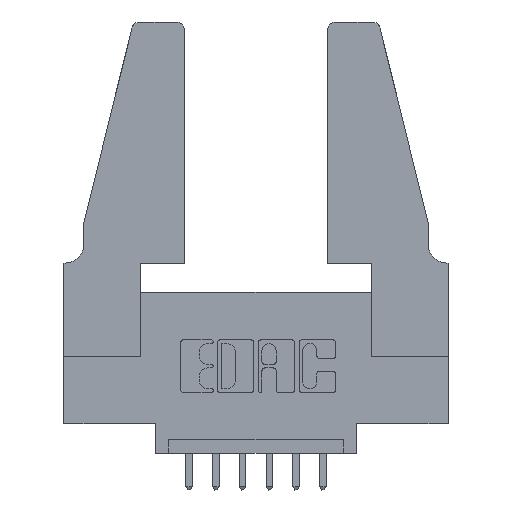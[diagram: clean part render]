
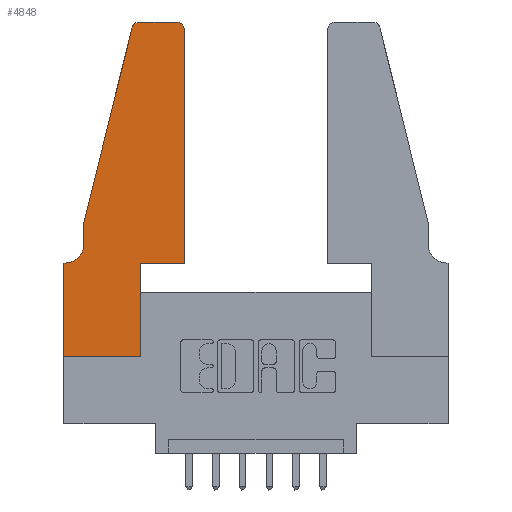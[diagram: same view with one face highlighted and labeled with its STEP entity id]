
A CAD part, top view. The second image highlights one B-rep face of the part: STEP entity #4848.
In plain terms, the highlighted planar face has unit normal (0, 0, 1).
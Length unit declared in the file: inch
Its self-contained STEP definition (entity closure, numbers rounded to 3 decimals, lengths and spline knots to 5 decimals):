
#144 = DIRECTION ( 'NONE',  ( 1., 0., 0. ) ) ;
#149 = VERTEX_POINT ( 'NONE', #6976 ) ;
#246 = ORIENTED_EDGE ( 'NONE', *, *, #10610, .T. ) ;
#506 = AXIS2_PLACEMENT_3D ( 'NONE', #6412, #2823, #144 ) ;
#513 = DIRECTION ( 'NONE',  ( -0.239, -0.971, 0. ) ) ;
#613 = LINE ( 'NONE', #10968, #7935 ) ;
#651 = EDGE_CURVE ( 'NONE', #149, #6248, #10727, .T. ) ;
#868 = AXIS2_PLACEMENT_3D ( 'NONE', #3825, #1192, #11094 ) ;
#982 = CARTESIAN_POINT ( 'NONE',  ( 0.4505, 1.22, 0.37 ) ) ;
#1148 = VERTEX_POINT ( 'NONE', #9154 ) ;
#1164 = VECTOR ( 'NONE', #2240, 39.37008 ) ;
#1192 = DIRECTION ( 'NONE',  ( 0., 0., -1. ) ) ;
#1407 = FACE_OUTER_BOUND ( 'NONE', #10970, .T. ) ;
#1627 = DIRECTION ( 'NONE',  ( 1., 0., 0. ) ) ;
#1780 = AXIS2_PLACEMENT_3D ( 'NONE', #10137, #6746, #8725 ) ;
#1840 = VECTOR ( 'NONE', #1627, 39.37008 ) ;
#2175 = LINE ( 'NONE', #9922, #9075 ) ;
#2212 = CARTESIAN_POINT ( 'NONE',  ( 0.0755, 0.42, 0.37 ) ) ;
#2240 = DIRECTION ( 'NONE',  ( 1., 0., 0. ) ) ;
#2250 = EDGE_CURVE ( 'NONE', #4102, #149, #9783, .T. ) ;
#2788 = EDGE_CURVE ( 'NONE', #1148, #4877, #2175, .T. ) ;
#2819 = VERTEX_POINT ( 'NONE', #5572 ) ;
#2823 = DIRECTION ( 'NONE',  ( 0., 0., 1. ) ) ;
#2910 = CARTESIAN_POINT ( 'NONE',  ( 0., 0.35, 0.37 ) ) ;
#2933 = EDGE_CURVE ( 'NONE', #4877, #8999, #613, .T. ) ;
#2944 = ORIENTED_EDGE ( 'NONE', *, *, #7547, .T. ) ;
#2983 = VERTEX_POINT ( 'NONE', #8595 ) ;
#3179 = CARTESIAN_POINT ( 'NONE',  ( 0.4505, 0.35, 0.37 ) ) ;
#3253 = CARTESIAN_POINT ( 'NONE',  ( 0.0755, 0.5, 0.37 ) ) ;
#3359 = EDGE_CURVE ( 'NONE', #10045, #2983, #6232, .T. ) ;
#3453 = VECTOR ( 'NONE', #9960, 39.37008 ) ;
#3467 = DIRECTION ( 'NONE',  ( -1., 0., 0. ) ) ;
#3476 = CARTESIAN_POINT ( 'NONE',  ( 0., 0., 0.37 ) ) ;
#3497 = ORIENTED_EDGE ( 'NONE', *, *, #5584, .T. ) ;
#3634 = VERTEX_POINT ( 'NONE', #6763 ) ;
#3640 = VERTEX_POINT ( 'NONE', #2212 ) ;
#3825 = CARTESIAN_POINT ( 'NONE',  ( 0.0055, 0.42, 0.37 ) ) ;
#3951 = ORIENTED_EDGE ( 'NONE', *, *, #651, .T. ) ;
#4093 = DIRECTION ( 'NONE',  ( 0., 1., 0. ) ) ;
#4102 = VERTEX_POINT ( 'NONE', #6157 ) ;
#4514 = DIRECTION ( 'NONE',  ( -1., 0., 0. ) ) ;
#4848 = ADVANCED_FACE ( 'NONE', ( #1407 ), #11075, .T. ) ;
#4877 = VERTEX_POINT ( 'NONE', #5651 ) ;
#4945 = EDGE_CURVE ( 'NONE', #6248, #3640, #10276, .T. ) ;
#5572 = CARTESIAN_POINT ( 'NONE',  ( 0.2865, 0., 0.37 ) ) ;
#5584 = EDGE_CURVE ( 'NONE', #2983, #4102, #9555, .T. ) ;
#5651 = CARTESIAN_POINT ( 'NONE',  ( 0., 0.35, 0.37 ) ) ;
#5797 = LINE ( 'NONE', #3179, #1164 ) ;
#5799 = DIRECTION ( 'NONE',  ( 0., -1., 0. ) ) ;
#6157 = CARTESIAN_POINT ( 'NONE',  ( 0.284, 1.25, 0.37 ) ) ;
#6232 = CIRCLE ( 'NONE', #506, 0.03 ) ;
#6248 = VERTEX_POINT ( 'NONE', #3253 ) ;
#6279 = CARTESIAN_POINT ( 'NONE',  ( 0.2865, 0.35, 0.37 ) ) ;
#6403 = LINE ( 'NONE', #6279, #3453 ) ;
#6412 = CARTESIAN_POINT ( 'NONE',  ( 0.4205, 1.22, 0.37 ) ) ;
#6470 = DIRECTION ( 'NONE',  ( 0., -1., 0. ) ) ;
#6471 = DIRECTION ( 'NONE',  ( 0., 0., 1. ) ) ;
#6548 = DIRECTION ( 'NONE',  ( 1., 0., 0. ) ) ;
#6746 = DIRECTION ( 'NONE',  ( 0., 0., 1. ) ) ;
#6763 = CARTESIAN_POINT ( 'NONE',  ( 0.4505, 0.35, 0.37 ) ) ;
#6843 = ORIENTED_EDGE ( 'NONE', *, *, #9702, .T. ) ;
#6976 = CARTESIAN_POINT ( 'NONE',  ( 0.25487, 1.22718, 0.37 ) ) ;
#7547 = EDGE_CURVE ( 'NONE', #2819, #9725, #6403, .T. ) ;
#7589 = VECTOR ( 'NONE', #5799, 39.37008 ) ;
#7645 = CARTESIAN_POINT ( 'NONE',  ( 0.4505, 0.35, 0.37 ) ) ;
#7740 = LINE ( 'NONE', #3476, #1840 ) ;
#7935 = VECTOR ( 'NONE', #6470, 39.37008 ) ;
#7981 = AXIS2_PLACEMENT_3D ( 'NONE', #2910, #6471, #6548 ) ;
#8316 = VECTOR ( 'NONE', #513, 39.37008 ) ;
#8525 = CARTESIAN_POINT ( 'NONE',  ( 0.2865, 0.35, 0.37 ) ) ;
#8572 = CARTESIAN_POINT ( 'NONE',  ( 0.0755, 0.5, 0.37 ) ) ;
#8594 = ORIENTED_EDGE ( 'NONE', *, *, #2788, .T. ) ;
#8595 = CARTESIAN_POINT ( 'NONE',  ( 0.4205, 1.25, 0.37 ) ) ;
#8596 = CARTESIAN_POINT ( 'NONE',  ( 0.0755, 0.5, 0.37 ) ) ;
#8725 = DIRECTION ( 'NONE',  ( 1., 0., 0. ) ) ;
#8810 = EDGE_CURVE ( 'NONE', #3640, #1148, #10909, .T. ) ;
#8827 = ORIENTED_EDGE ( 'NONE', *, *, #10438, .T. ) ;
#8850 = CARTESIAN_POINT ( 'NONE',  ( 0.2605, 1.25, 0.37 ) ) ;
#8999 = VERTEX_POINT ( 'NONE', #11297 ) ;
#9001 = VECTOR ( 'NONE', #3467, 39.37008 ) ;
#9057 = ORIENTED_EDGE ( 'NONE', *, *, #8810, .T. ) ;
#9075 = VECTOR ( 'NONE', #4514, 39.37008 ) ;
#9082 = ORIENTED_EDGE ( 'NONE', *, *, #2250, .T. ) ;
#9126 = ORIENTED_EDGE ( 'NONE', *, *, #2933, .T. ) ;
#9154 = CARTESIAN_POINT ( 'NONE',  ( 0.0055, 0.35, 0.37 ) ) ;
#9555 = LINE ( 'NONE', #8850, #9001 ) ;
#9702 = EDGE_CURVE ( 'NONE', #9725, #3634, #5797, .T. ) ;
#9725 = VERTEX_POINT ( 'NONE', #8525 ) ;
#9726 = LINE ( 'NONE', #7645, #10169 ) ;
#9783 = CIRCLE ( 'NONE', #1780, 0.03 ) ;
#9922 = CARTESIAN_POINT ( 'NONE',  ( 0.0755, 0.35, 0.37 ) ) ;
#9960 = DIRECTION ( 'NONE',  ( 0., 1., 0. ) ) ;
#10045 = VERTEX_POINT ( 'NONE', #982 ) ;
#10137 = CARTESIAN_POINT ( 'NONE',  ( 0.284, 1.22, 0.37 ) ) ;
#10169 = VECTOR ( 'NONE', #4093, 39.37008 ) ;
#10276 = LINE ( 'NONE', #8596, #7589 ) ;
#10438 = EDGE_CURVE ( 'NONE', #3634, #10045, #9726, .T. ) ;
#10592 = ORIENTED_EDGE ( 'NONE', *, *, #4945, .T. ) ;
#10610 = EDGE_CURVE ( 'NONE', #8999, #2819, #7740, .T. ) ;
#10727 = LINE ( 'NONE', #8572, #8316 ) ;
#10909 = CIRCLE ( 'NONE', #868, 0.07 ) ;
#10968 = CARTESIAN_POINT ( 'NONE',  ( 0., 0., 0.37 ) ) ;
#10970 = EDGE_LOOP ( 'NONE', ( #3497, #9082, #3951, #10592, #9057, #8594, #9126, #246, #2944, #6843, #8827, #11595 ) ) ;
#11075 = PLANE ( 'NONE',  #7981 ) ;
#11094 = DIRECTION ( 'NONE',  ( -1., 0., 0. ) ) ;
#11297 = CARTESIAN_POINT ( 'NONE',  ( 0., 0., 0.37 ) ) ;
#11595 = ORIENTED_EDGE ( 'NONE', *, *, #3359, .T. ) ;
